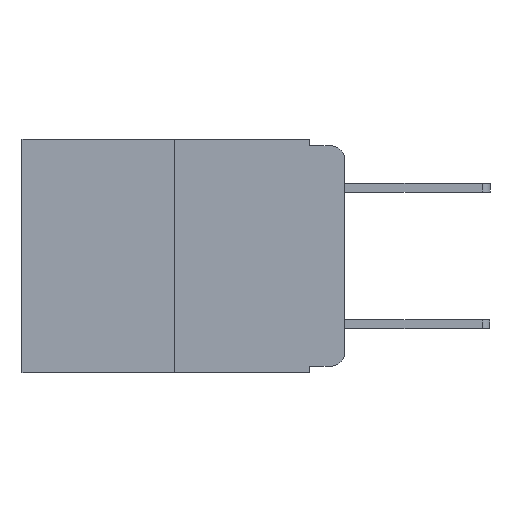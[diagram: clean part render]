
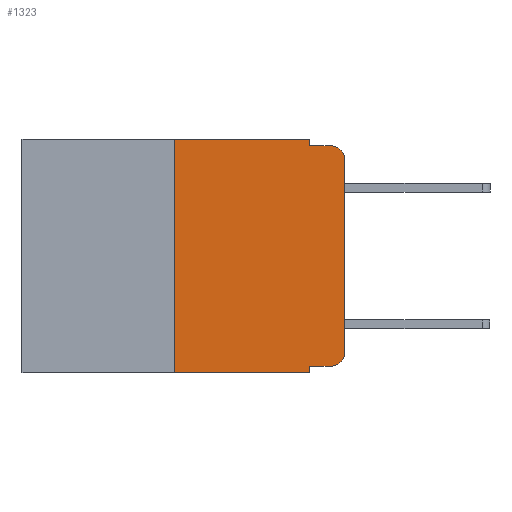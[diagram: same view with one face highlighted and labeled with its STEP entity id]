
A CAD part, left-side view. The second image highlights one B-rep face of the part: STEP entity #1323.
In plain terms, the highlighted planar face has unit normal (-1, 0, 0).
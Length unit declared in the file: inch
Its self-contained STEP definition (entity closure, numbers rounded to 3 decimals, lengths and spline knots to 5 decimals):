
#69 = EDGE_CURVE ( 'NONE', #9155, #19451, #18397, .T. ) ;
#526 = LINE ( 'NONE', #15968, #16653 ) ;
#861 = VECTOR ( 'NONE', #8655, 39.37008 ) ;
#862 = VERTEX_POINT ( 'NONE', #16801 ) ;
#963 = DIRECTION ( 'NONE',  ( -1., 0., 0. ) ) ;
#1237 = EDGE_CURVE ( 'NONE', #5901, #11154, #4709, .T. ) ;
#1323 = ADVANCED_FACE ( 'NONE', ( #2752 ), #18302, .F. ) ;
#1415 = VECTOR ( 'NONE', #17110, 39.37008 ) ;
#1550 = EDGE_CURVE ( 'NONE', #5901, #19451, #4688, .T. ) ;
#1942 = ORIENTED_EDGE ( 'NONE', *, *, #18222, .T. ) ;
#2432 = EDGE_CURVE ( 'NONE', #862, #3562, #526, .T. ) ;
#2700 = ORIENTED_EDGE ( 'NONE', *, *, #6615, .T. ) ;
#2752 = FACE_OUTER_BOUND ( 'NONE', #7456, .T. ) ;
#3029 = VERTEX_POINT ( 'NONE', #11814 ) ;
#3150 = CARTESIAN_POINT ( 'NONE',  ( 0., 0., 0. ) ) ;
#3489 = EDGE_CURVE ( 'NONE', #3562, #3029, #17216, .T. ) ;
#3562 = VERTEX_POINT ( 'NONE', #18271 ) ;
#3635 = DIRECTION ( 'NONE',  ( 1., 0., 0. ) ) ;
#3675 = DIRECTION ( 'NONE',  ( 0., 0., -1. ) ) ;
#4688 = LINE ( 'NONE', #9480, #861 ) ;
#4709 = LINE ( 'NONE', #12512, #5682 ) ;
#5149 = ORIENTED_EDGE ( 'NONE', *, *, #69, .F. ) ;
#5682 = VECTOR ( 'NONE', #12517, 39.37008 ) ;
#5901 = VERTEX_POINT ( 'NONE', #18012 ) ;
#5960 = CARTESIAN_POINT ( 'NONE',  ( 0., 0.02, -0.03 ) ) ;
#6370 = ORIENTED_EDGE ( 'NONE', *, *, #7621, .T. ) ;
#6581 = VECTOR ( 'NONE', #9376, 39.37008 ) ;
#6615 = EDGE_CURVE ( 'NONE', #7513, #3029, #19614, .T. ) ;
#7301 = ORIENTED_EDGE ( 'NONE', *, *, #2432, .F. ) ;
#7379 = CARTESIAN_POINT ( 'NONE',  ( 0., 0., -0.313 ) ) ;
#7456 = EDGE_LOOP ( 'NONE', ( #6370, #2700, #18957, #7301, #8306, #16447, #16901, #5149, #17370, #1942 ) ) ;
#7501 = DIRECTION ( 'NONE',  ( 0., 0., -1. ) ) ;
#7513 = VERTEX_POINT ( 'NONE', #13039 ) ;
#7621 = EDGE_CURVE ( 'NONE', #14013, #7513, #14747, .T. ) ;
#8217 = DIRECTION ( 'NONE',  ( 0., -1., 0. ) ) ;
#8306 = ORIENTED_EDGE ( 'NONE', *, *, #19661, .F. ) ;
#8655 = DIRECTION ( 'NONE',  ( 0., -1., 0. ) ) ;
#9155 = VERTEX_POINT ( 'NONE', #17513 ) ;
#9305 = VECTOR ( 'NONE', #18459, 39.37008 ) ;
#9376 = DIRECTION ( 'NONE',  ( 0., 0., 1. ) ) ;
#9381 = CARTESIAN_POINT ( 'NONE',  ( 0., 0.473, 0. ) ) ;
#9480 = CARTESIAN_POINT ( 'NONE',  ( 0., 0.473, -0.343 ) ) ;
#9810 = LINE ( 'NONE', #11084, #1415 ) ;
#9970 = AXIS2_PLACEMENT_3D ( 'NONE', #10432, #963, #11972 ) ;
#10362 = CARTESIAN_POINT ( 'NONE',  ( 0., 0.051, -0.01 ) ) ;
#10432 = CARTESIAN_POINT ( 'NONE',  ( 0., 0.02, -0.313 ) ) ;
#10454 = CARTESIAN_POINT ( 'NONE',  ( 0., 0.051, -0.343 ) ) ;
#10825 = VECTOR ( 'NONE', #19517, 39.37008 ) ;
#11084 = CARTESIAN_POINT ( 'NONE',  ( 0., 0.051, -0.333 ) ) ;
#11154 = VERTEX_POINT ( 'NONE', #13375 ) ;
#11814 = CARTESIAN_POINT ( 'NONE',  ( 0., 0.02, -0.01 ) ) ;
#11972 = DIRECTION ( 'NONE',  ( 0., 0., -1. ) ) ;
#12512 = CARTESIAN_POINT ( 'NONE',  ( 0., 0.25, 0. ) ) ;
#12517 = DIRECTION ( 'NONE',  ( 0., 0., 1. ) ) ;
#12524 = AXIS2_PLACEMENT_3D ( 'NONE', #13399, #3635, #3675 ) ;
#12812 = AXIS2_PLACEMENT_3D ( 'NONE', #5960, #16690, #7501 ) ;
#13039 = CARTESIAN_POINT ( 'NONE',  ( 0., 0., -0.03 ) ) ;
#13219 = VECTOR ( 'NONE', #8217, 39.37008 ) ;
#13375 = CARTESIAN_POINT ( 'NONE',  ( 0., 0.25, 0. ) ) ;
#13399 = CARTESIAN_POINT ( 'NONE',  ( 0., 0.473, 0. ) ) ;
#13498 = DIRECTION ( 'NONE',  ( 0., 0., -1. ) ) ;
#14013 = VERTEX_POINT ( 'NONE', #7379 ) ;
#14747 = LINE ( 'NONE', #3150, #6581 ) ;
#15957 = CARTESIAN_POINT ( 'NONE',  ( 0., 0.02, -0.333 ) ) ;
#15968 = CARTESIAN_POINT ( 'NONE',  ( 0., 0.051, 0. ) ) ;
#16447 = ORIENTED_EDGE ( 'NONE', *, *, #1237, .F. ) ;
#16653 = VECTOR ( 'NONE', #13498, 39.37008 ) ;
#16690 = DIRECTION ( 'NONE',  ( -1., 0., 0. ) ) ;
#16801 = CARTESIAN_POINT ( 'NONE',  ( 0., 0.051, 0. ) ) ;
#16901 = ORIENTED_EDGE ( 'NONE', *, *, #1550, .T. ) ;
#17110 = DIRECTION ( 'NONE',  ( 0., -1., 0. ) ) ;
#17216 = LINE ( 'NONE', #10362, #13219 ) ;
#17370 = ORIENTED_EDGE ( 'NONE', *, *, #19177, .T. ) ;
#17513 = CARTESIAN_POINT ( 'NONE',  ( 0., 0.051, -0.333 ) ) ;
#17855 = LINE ( 'NONE', #9381, #9305 ) ;
#17893 = CARTESIAN_POINT ( 'NONE',  ( 0., 0.051, 0. ) ) ;
#17914 = CIRCLE ( 'NONE', #9970, 0.02 ) ;
#17978 = VERTEX_POINT ( 'NONE', #15957 ) ;
#18012 = CARTESIAN_POINT ( 'NONE',  ( 0., 0.25, -0.343 ) ) ;
#18222 = EDGE_CURVE ( 'NONE', #17978, #14013, #17914, .T. ) ;
#18271 = CARTESIAN_POINT ( 'NONE',  ( 0., 0.051, -0.01 ) ) ;
#18302 = PLANE ( 'NONE',  #12524 ) ;
#18397 = LINE ( 'NONE', #17893, #10825 ) ;
#18459 = DIRECTION ( 'NONE',  ( 0., -1., 0. ) ) ;
#18957 = ORIENTED_EDGE ( 'NONE', *, *, #3489, .F. ) ;
#19177 = EDGE_CURVE ( 'NONE', #9155, #17978, #9810, .T. ) ;
#19451 = VERTEX_POINT ( 'NONE', #10454 ) ;
#19517 = DIRECTION ( 'NONE',  ( 0., 0., -1. ) ) ;
#19614 = CIRCLE ( 'NONE', #12812, 0.02 ) ;
#19661 = EDGE_CURVE ( 'NONE', #11154, #862, #17855, .T. ) ;
